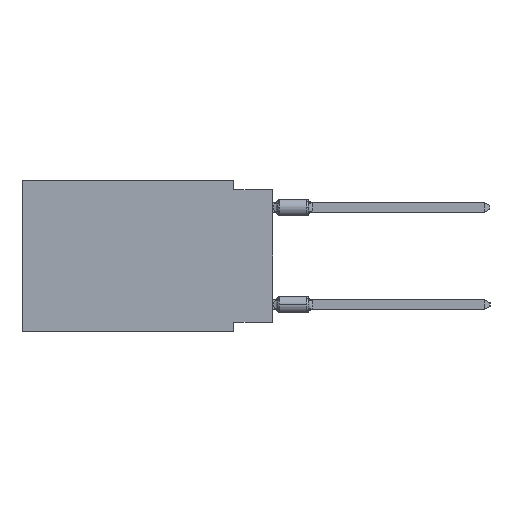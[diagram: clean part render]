
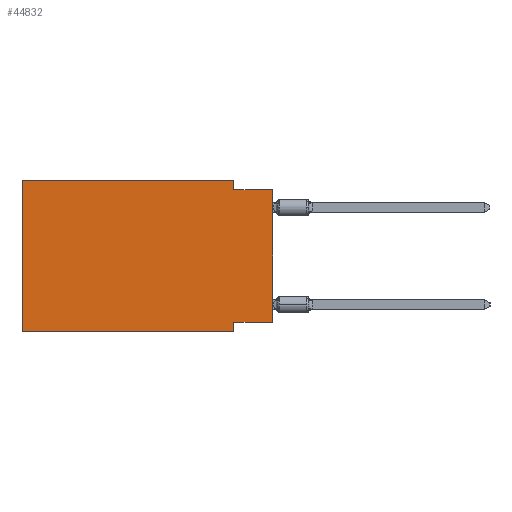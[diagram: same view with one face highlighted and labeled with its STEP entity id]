
A CAD part, left-side view. The second image highlights one B-rep face of the part: STEP entity #44832.
In plain terms, the highlighted planar face has unit normal (-1, 0, 0).
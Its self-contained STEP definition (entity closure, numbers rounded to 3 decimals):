
#1932 = ORIENTED_EDGE ( 'NONE', *, *, #7270, .F. ) ;
#2183 = LINE ( 'NONE', #7113, #44515 ) ;
#2335 = CARTESIAN_POINT ( 'NONE',  ( 0., 2.54, -9.906 ) ) ;
#2630 = ORIENTED_EDGE ( 'NONE', *, *, #3514, .F. ) ;
#3457 = LINE ( 'NONE', #48191, #44943 ) ;
#3514 = EDGE_CURVE ( 'NONE', #19024, #52853, #56471, .T. ) ;
#4655 = CARTESIAN_POINT ( 'NONE',  ( 0., 2.54, 0. ) ) ;
#5539 = EDGE_CURVE ( 'NONE', #44936, #10199, #29123, .T. ) ;
#6104 = PLANE ( 'NONE',  #41172 ) ;
#7113 = CARTESIAN_POINT ( 'NONE',  ( 0., 2.54, -9.906 ) ) ;
#7235 = CARTESIAN_POINT ( 'NONE',  ( 0., 0., -9.271 ) ) ;
#7270 = EDGE_CURVE ( 'NONE', #52013, #25258, #20699, .T. ) ;
#9184 = LINE ( 'NONE', #27008, #48547 ) ;
#10007 = CARTESIAN_POINT ( 'NONE',  ( 0., 2.54, -0.635 ) ) ;
#10199 = VERTEX_POINT ( 'NONE', #2335 ) ;
#10790 = DIRECTION ( 'NONE',  ( 0., 0., -1. ) ) ;
#10859 = CARTESIAN_POINT ( 'NONE',  ( 0., 16.383, 0. ) ) ;
#10907 = EDGE_CURVE ( 'NONE', #19855, #30203, #9184, .T. ) ;
#12452 = VECTOR ( 'NONE', #19950, 1000. ) ;
#12921 = ORIENTED_EDGE ( 'NONE', *, *, #5539, .T. ) ;
#13600 = EDGE_CURVE ( 'NONE', #52013, #30203, #45702, .T. ) ;
#15165 = CARTESIAN_POINT ( 'NONE',  ( 0., 16.383, 0. ) ) ;
#17156 = ORIENTED_EDGE ( 'NONE', *, *, #44839, .F. ) ;
#18813 = DIRECTION ( 'NONE',  ( 0., -1., 0. ) ) ;
#19024 = VERTEX_POINT ( 'NONE', #35965 ) ;
#19855 = VERTEX_POINT ( 'NONE', #10007 ) ;
#19950 = DIRECTION ( 'NONE',  ( 0., 0., 1. ) ) ;
#20003 = DIRECTION ( 'NONE',  ( 0., 0., -1. ) ) ;
#20699 = LINE ( 'NONE', #7235, #37874 ) ;
#22450 = CARTESIAN_POINT ( 'NONE',  ( 0., 16.383, -9.906 ) ) ;
#23182 = CARTESIAN_POINT ( 'NONE',  ( 0., 0., -9.271 ) ) ;
#25258 = VERTEX_POINT ( 'NONE', #50786 ) ;
#27008 = CARTESIAN_POINT ( 'NONE',  ( 0., 0., -0.635 ) ) ;
#27447 = DIRECTION ( 'NONE',  ( 0., 0., 1. ) ) ;
#28317 = FACE_OUTER_BOUND ( 'NONE', #30180, .T. ) ;
#29123 = LINE ( 'NONE', #37899, #52870 ) ;
#29826 = DIRECTION ( 'NONE',  ( 0., -1., 0. ) ) ;
#30180 = EDGE_LOOP ( 'NONE', ( #32327, #45824, #17156, #2630, #34702, #12921, #38130, #1932 ) ) ;
#30203 = VERTEX_POINT ( 'NONE', #51807 ) ;
#32327 = ORIENTED_EDGE ( 'NONE', *, *, #13600, .T. ) ;
#33015 = DIRECTION ( 'NONE',  ( 1., 0., 0. ) ) ;
#34702 = ORIENTED_EDGE ( 'NONE', *, *, #52875, .F. ) ;
#35348 = LINE ( 'NONE', #49104, #47297 ) ;
#35965 = CARTESIAN_POINT ( 'NONE',  ( 0., 16.383, 0. ) ) ;
#37874 = VECTOR ( 'NONE', #51730, 1000. ) ;
#37899 = CARTESIAN_POINT ( 'NONE',  ( 0., 16.383, -9.906 ) ) ;
#38130 = ORIENTED_EDGE ( 'NONE', *, *, #39922, .F. ) ;
#38180 = DIRECTION ( 'NONE',  ( 0., -1., 0. ) ) ;
#39922 = EDGE_CURVE ( 'NONE', #25258, #10199, #2183, .T. ) ;
#41172 = AXIS2_PLACEMENT_3D ( 'NONE', #15165, #33015, #10790 ) ;
#44515 = VECTOR ( 'NONE', #20003, 1000. ) ;
#44832 = ADVANCED_FACE ( 'NONE', ( #28317 ), #6104, .F. ) ;
#44839 = EDGE_CURVE ( 'NONE', #52853, #19855, #3457, .T. ) ;
#44936 = VERTEX_POINT ( 'NONE', #22450 ) ;
#44943 = VECTOR ( 'NONE', #48769, 1000. ) ;
#45702 = LINE ( 'NONE', #46555, #12452 ) ;
#45824 = ORIENTED_EDGE ( 'NONE', *, *, #10907, .F. ) ;
#46555 = CARTESIAN_POINT ( 'NONE',  ( 0., 0., 0. ) ) ;
#47297 = VECTOR ( 'NONE', #27447, 1000. ) ;
#48191 = CARTESIAN_POINT ( 'NONE',  ( 0., 2.54, 0. ) ) ;
#48547 = VECTOR ( 'NONE', #18813, 1000. ) ;
#48769 = DIRECTION ( 'NONE',  ( 0., 0., -1. ) ) ;
#49104 = CARTESIAN_POINT ( 'NONE',  ( 0., 16.383, 0. ) ) ;
#49801 = VECTOR ( 'NONE', #29826, 1000. ) ;
#50786 = CARTESIAN_POINT ( 'NONE',  ( 0., 2.54, -9.271 ) ) ;
#51730 = DIRECTION ( 'NONE',  ( 0., 1., 0. ) ) ;
#51807 = CARTESIAN_POINT ( 'NONE',  ( 0., 0., -0.635 ) ) ;
#52013 = VERTEX_POINT ( 'NONE', #23182 ) ;
#52853 = VERTEX_POINT ( 'NONE', #4655 ) ;
#52870 = VECTOR ( 'NONE', #38180, 1000. ) ;
#52875 = EDGE_CURVE ( 'NONE', #44936, #19024, #35348, .T. ) ;
#56471 = LINE ( 'NONE', #10859, #49801 ) ;
